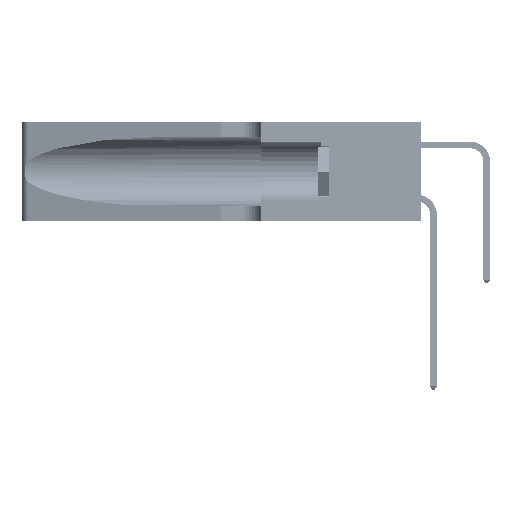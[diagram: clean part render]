
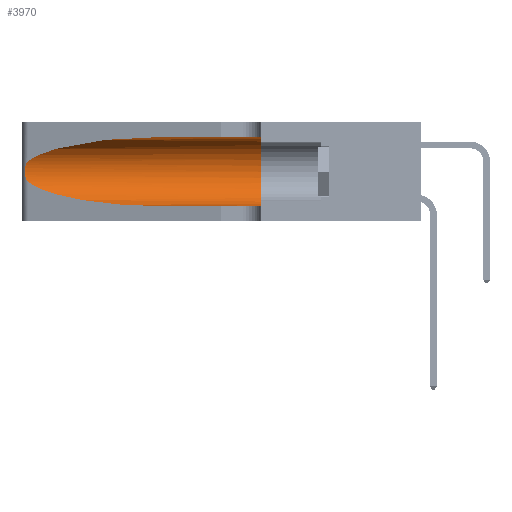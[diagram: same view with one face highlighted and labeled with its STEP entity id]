
A CAD part, left-side view. The second image highlights one B-rep face of the part: STEP entity #3970.
In plain terms, the highlighted cylindrical face has radius 3.308 mm (diameter 6.617 mm), a partial arc.
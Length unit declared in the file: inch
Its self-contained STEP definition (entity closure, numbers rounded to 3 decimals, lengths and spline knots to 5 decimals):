
#151 = CARTESIAN_POINT ( 'NONE',  ( 0.25487, 1.22718, 0.14631 ) ) ;
#647 = CARTESIAN_POINT ( 'NONE',  ( 0.2373, 1.15595, 0.08982 ) ) ;
#1219 = DIRECTION ( 'NONE',  ( 0., -1., 0. ) ) ;
#2232 = EDGE_CURVE ( 'NONE', #7661, #15655, #3356, .T. ) ;
#2739 = CARTESIAN_POINT ( 'NONE',  ( 0.26075, 1.23896, 0.19203 ) ) ;
#3356 = B_SPLINE_CURVE_WITH_KNOTS ( 'NONE', 3,
 ( #21559, #10026, #13910, #14734, #30113, #11187, #2739, #22572, #49419, #14903, #41569, #6814, #26009, #29956 ),
 .UNSPECIFIED., .F., .F.,
 ( 4, 2, 2, 2, 2, 2, 4 ),
 ( 0., 0.00027, 0.00053, 0.00107, 0.0016, 0.00187, 0.00214 ),
 .UNSPECIFIED. ) ;
#3970 = ADVANCED_FACE ( 'NONE', ( #36778 ), #47835, .F. ) ;
#5821 = CARTESIAN_POINT ( 'NONE',  ( 0.1305, 1.61858, 0.05475 ) ) ;
#6814 = CARTESIAN_POINT ( 'NONE',  ( 0.25639, 1.23186, 0.15144 ) ) ;
#7093 =( BOUNDED_CURVE ( )  B_SPLINE_CURVE ( 3, ( #26102, #14332, #10780, #21982 ),
 .UNSPECIFIED., .F., .F. ) 
 B_SPLINE_CURVE_WITH_KNOTS ( ( 4, 4 ),
 ( 1.5708, 2.84003 ),
 .UNSPECIFIED. ) 
 CURVE ( )  GEOMETRIC_REPRESENTATION_ITEM ( )  RATIONAL_B_SPLINE_CURVE ( ( 1., 0.87, 0.87, 1. ) ) 
 REPRESENTATION_ITEM ( '' )  );
#7404 = ORIENTED_EDGE ( 'NONE', *, *, #13434, .T. ) ;
#7661 = VERTEX_POINT ( 'NONE', #48864 ) ;
#8703 = CARTESIAN_POINT ( 'NONE',  ( 0.1305, 0.72297, 0.31525 ) ) ;
#10000 = EDGE_CURVE ( 'NONE', #27321, #26831, #17193, .T. ) ;
#10026 = CARTESIAN_POINT ( 'NONE',  ( 0.25555, 1.22994, 0.2215 ) ) ;
#10780 = CARTESIAN_POINT ( 'NONE',  ( 0.2373, 1.15595, 0.28018 ) ) ;
#11187 = CARTESIAN_POINT ( 'NONE',  ( 0.26018, 1.23835, 0.19895 ) ) ;
#12258 = CARTESIAN_POINT ( 'NONE',  ( 0.25487, 1.22718, 0.14631 ) ) ;
#13434 = EDGE_CURVE ( 'NONE', #15655, #27321, #37990, .T. ) ;
#13910 = CARTESIAN_POINT ( 'NONE',  ( 0.25639, 1.23184, 0.21858 ) ) ;
#14256 = CIRCLE ( 'NONE', #35932, 0.13025 ) ;
#14332 = CARTESIAN_POINT ( 'NONE',  ( 0.18966, 0.96281, 0.31525 ) ) ;
#14341 = VECTOR ( 'NONE', #33559, 39.37008 ) ;
#14734 = CARTESIAN_POINT ( 'NONE',  ( 0.25787, 1.23484, 0.2124 ) ) ;
#14903 = CARTESIAN_POINT ( 'NONE',  ( 0.25856, 1.23593, 0.16098 ) ) ;
#15655 = VERTEX_POINT ( 'NONE', #12258 ) ;
#17193 = LINE ( 'NONE', #5821, #19640 ) ;
#19640 = VECTOR ( 'NONE', #43972, 39.37008 ) ;
#19725 = CARTESIAN_POINT ( 'NONE',  ( 0.1305, 0.35, 0.185 ) ) ;
#21475 = CARTESIAN_POINT ( 'NONE',  ( 0.1305, 0.72297, 0.05475 ) ) ;
#21559 = CARTESIAN_POINT ( 'NONE',  ( 0.25487, 1.22718, 0.22369 ) ) ;
#21982 = CARTESIAN_POINT ( 'NONE',  ( 0.25487, 1.22718, 0.22369 ) ) ;
#22572 = CARTESIAN_POINT ( 'NONE',  ( 0.26075, 1.23896, 0.178 ) ) ;
#24725 = ORIENTED_EDGE ( 'NONE', *, *, #34427, .F. ) ;
#24817 = CARTESIAN_POINT ( 'NONE',  ( 0.1305, 1.61858, 0.185 ) ) ;
#25876 = EDGE_CURVE ( 'NONE', #36564, #7661, #7093, .T. ) ;
#26009 = CARTESIAN_POINT ( 'NONE',  ( 0.25555, 1.22993, 0.14849 ) ) ;
#26102 = CARTESIAN_POINT ( 'NONE',  ( 0.1305, 0.72297, 0.31525 ) ) ;
#26831 = VERTEX_POINT ( 'NONE', #41357 ) ;
#27321 = VERTEX_POINT ( 'NONE', #21475 ) ;
#27702 = ORIENTED_EDGE ( 'NONE', *, *, #43551, .F. ) ;
#29255 = AXIS2_PLACEMENT_3D ( 'NONE', #24817, #1219, #36430 ) ;
#29637 = CARTESIAN_POINT ( 'NONE',  ( 0.1305, 1.61858, 0.31525 ) ) ;
#29755 = ORIENTED_EDGE ( 'NONE', *, *, #10000, .T. ) ;
#29956 = CARTESIAN_POINT ( 'NONE',  ( 0.25487, 1.22718, 0.14631 ) ) ;
#30113 = CARTESIAN_POINT ( 'NONE',  ( 0.25854, 1.2359, 0.20912 ) ) ;
#30507 = CARTESIAN_POINT ( 'NONE',  ( 0.1305, 0.35, 0.31525 ) ) ;
#33559 = DIRECTION ( 'NONE',  ( 0., -1., 0. ) ) ;
#34427 = EDGE_CURVE ( 'NONE', #36564, #48709, #45498, .T. ) ;
#35455 = DIRECTION ( 'NONE',  ( 0., 0., 1. ) ) ;
#35932 = AXIS2_PLACEMENT_3D ( 'NONE', #19725, #47401, #35455 ) ;
#36430 = DIRECTION ( 'NONE',  ( 0., 0., -1. ) ) ;
#36564 = VERTEX_POINT ( 'NONE', #8703 ) ;
#36778 = FACE_OUTER_BOUND ( 'NONE', #40525, .T. ) ;
#37066 = ORIENTED_EDGE ( 'NONE', *, *, #25876, .T. ) ;
#37593 = ORIENTED_EDGE ( 'NONE', *, *, #2232, .T. ) ;
#37990 =( BOUNDED_CURVE ( )  B_SPLINE_CURVE ( 3, ( #151, #647, #39110, #39454 ),
 .UNSPECIFIED., .F., .F. ) 
 B_SPLINE_CURVE_WITH_KNOTS ( ( 4, 4 ),
 ( 3.44316, 4.71239 ),
 .UNSPECIFIED. ) 
 CURVE ( )  GEOMETRIC_REPRESENTATION_ITEM ( )  RATIONAL_B_SPLINE_CURVE ( ( 1., 0.87, 0.87, 1. ) ) 
 REPRESENTATION_ITEM ( '' )  );
#39110 = CARTESIAN_POINT ( 'NONE',  ( 0.18966, 0.96281, 0.05475 ) ) ;
#39454 = CARTESIAN_POINT ( 'NONE',  ( 0.1305, 0.72297, 0.05475 ) ) ;
#40525 = EDGE_LOOP ( 'NONE', ( #37066, #37593, #7404, #29755, #27702, #24725 ) ) ;
#41357 = CARTESIAN_POINT ( 'NONE',  ( 0.1305, 0.35, 0.05475 ) ) ;
#41569 = CARTESIAN_POINT ( 'NONE',  ( 0.25789, 1.23486, 0.15765 ) ) ;
#43551 = EDGE_CURVE ( 'NONE', #48709, #26831, #14256, .T. ) ;
#43972 = DIRECTION ( 'NONE',  ( 0., -1., 0. ) ) ;
#45498 = LINE ( 'NONE', #29637, #14341 ) ;
#47401 = DIRECTION ( 'NONE',  ( 0., 1., 0. ) ) ;
#47835 = CYLINDRICAL_SURFACE ( 'NONE', #29255, 0.13025 ) ;
#48709 = VERTEX_POINT ( 'NONE', #30507 ) ;
#48864 = CARTESIAN_POINT ( 'NONE',  ( 0.25487, 1.22718, 0.22369 ) ) ;
#49419 = CARTESIAN_POINT ( 'NONE',  ( 0.26017, 1.23833, 0.17102 ) ) ;
